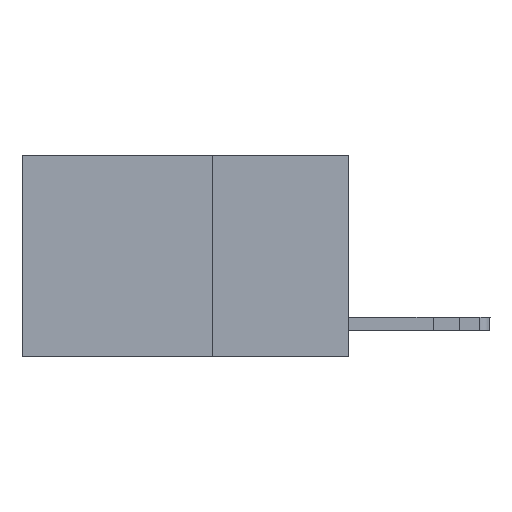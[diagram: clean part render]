
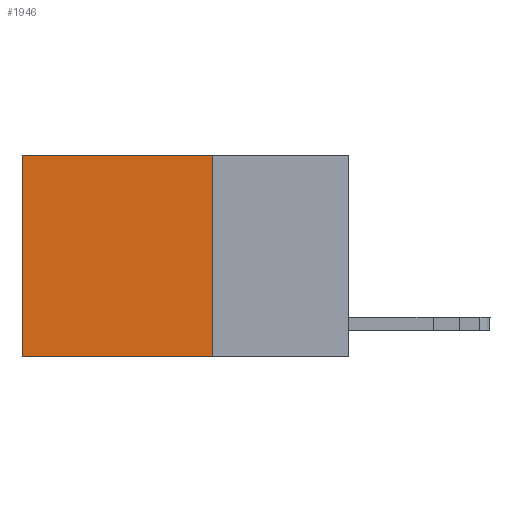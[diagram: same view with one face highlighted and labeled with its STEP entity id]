
A CAD part, left-side view. The second image highlights one B-rep face of the part: STEP entity #1946.
In plain terms, the highlighted planar face has unit normal (-1, 0, 0).
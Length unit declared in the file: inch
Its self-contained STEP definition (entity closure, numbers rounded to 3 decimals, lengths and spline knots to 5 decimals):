
#23 = DIRECTION ( 'NONE',  ( 0., 1., 0. ) ) ;
#1129 = LINE ( 'NONE', #3521, #4128 ) ;
#1563 = CARTESIAN_POINT ( 'NONE',  ( 0.2625, 0.25, 0. ) ) ;
#1778 = VECTOR ( 'NONE', #23, 39.37008 ) ;
#1946 = ADVANCED_FACE ( 'NONE', ( #13652 ), #14870, .F. ) ;
#2251 = CARTESIAN_POINT ( 'NONE',  ( 0.2625, 0.25, -0.37 ) ) ;
#3521 = CARTESIAN_POINT ( 'NONE',  ( 0.2625, 0.25, 0. ) ) ;
#3764 = CARTESIAN_POINT ( 'NONE',  ( 0.2625, 0.25, 0. ) ) ;
#3952 = DIRECTION ( 'NONE',  ( 1., 0., 0. ) ) ;
#3987 = DIRECTION ( 'NONE',  ( 0., 1., 0. ) ) ;
#4039 = EDGE_CURVE ( 'NONE', #5798, #8345, #5895, .T. ) ;
#4128 = VECTOR ( 'NONE', #5741, 39.37008 ) ;
#4207 = CARTESIAN_POINT ( 'NONE',  ( 0.2625, 0.25, 0. ) ) ;
#5040 = EDGE_CURVE ( 'NONE', #8345, #14810, #8008, .T. ) ;
#5375 = ORIENTED_EDGE ( 'NONE', *, *, #5040, .T. ) ;
#5383 = EDGE_CURVE ( 'NONE', #6529, #14810, #6443, .T. ) ;
#5741 = DIRECTION ( 'NONE',  ( 0., 0., -1. ) ) ;
#5798 = VERTEX_POINT ( 'NONE', #4207 ) ;
#5803 = VECTOR ( 'NONE', #11499, 39.37008 ) ;
#5895 = LINE ( 'NONE', #3764, #1778 ) ;
#6443 = LINE ( 'NONE', #7555, #14478 ) ;
#6529 = VERTEX_POINT ( 'NONE', #2251 ) ;
#7555 = CARTESIAN_POINT ( 'NONE',  ( 0.2625, 0.25, -0.37 ) ) ;
#7841 = CARTESIAN_POINT ( 'NONE',  ( 0.2625, 0.6, -0.37 ) ) ;
#8008 = LINE ( 'NONE', #15344, #5803 ) ;
#8345 = VERTEX_POINT ( 'NONE', #13154 ) ;
#8490 = AXIS2_PLACEMENT_3D ( 'NONE', #1563, #3952, #8793 ) ;
#8793 = DIRECTION ( 'NONE',  ( 0., 0., -1. ) ) ;
#10409 = EDGE_CURVE ( 'NONE', #5798, #6529, #1129, .T. ) ;
#11499 = DIRECTION ( 'NONE',  ( 0., 0., -1. ) ) ;
#11924 = EDGE_LOOP ( 'NONE', ( #5375, #15230, #14740, #12568 ) ) ;
#12568 = ORIENTED_EDGE ( 'NONE', *, *, #4039, .T. ) ;
#13154 = CARTESIAN_POINT ( 'NONE',  ( 0.2625, 0.6, 0. ) ) ;
#13652 = FACE_OUTER_BOUND ( 'NONE', #11924, .T. ) ;
#14478 = VECTOR ( 'NONE', #3987, 39.37008 ) ;
#14740 = ORIENTED_EDGE ( 'NONE', *, *, #10409, .F. ) ;
#14810 = VERTEX_POINT ( 'NONE', #7841 ) ;
#14870 = PLANE ( 'NONE',  #8490 ) ;
#15230 = ORIENTED_EDGE ( 'NONE', *, *, #5383, .F. ) ;
#15344 = CARTESIAN_POINT ( 'NONE',  ( 0.2625, 0.6, 0. ) ) ;
